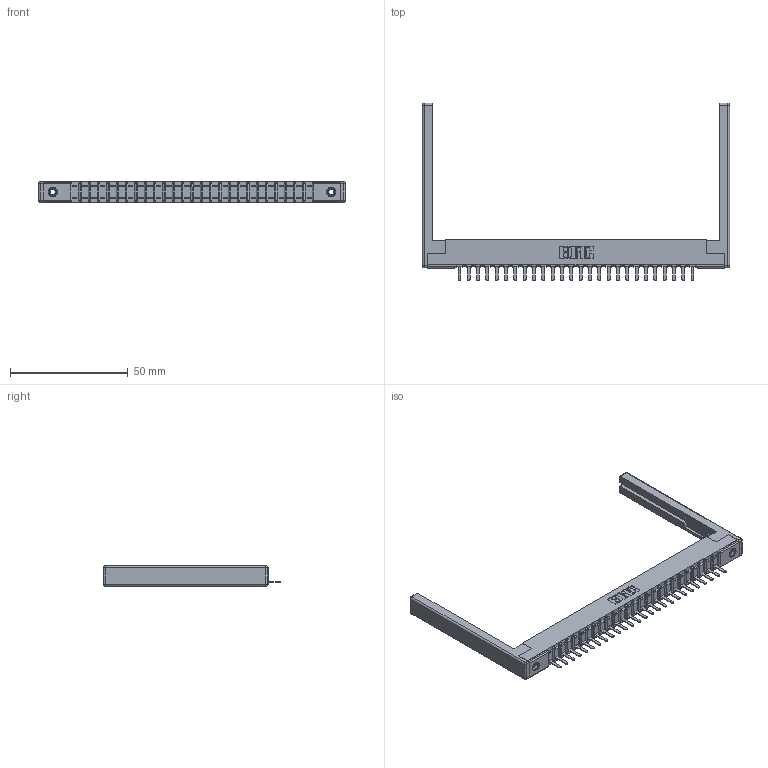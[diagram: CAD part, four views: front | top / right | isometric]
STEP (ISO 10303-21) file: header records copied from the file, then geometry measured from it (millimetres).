
FILE_DESCRIPTION (( 'STEP AP203' ), '1' );
FILE_NAME ('357-026-521-168.STEP', '2019-09-17T01:04:23', ( '' ), ( '' ), 'SwSTEP 2.0', 'SolidWorks 2016', '' );
FILE_SCHEMA (( 'CONFIG_CONTROL_DESIGN' ));
Length unit declared in the file: inch
Products named in the file (5): 307-290-002_521; 307 Part_.156 Dia Mounting Holes; 357-026-521-168; 307-220-068; 345-250-001_345-250-001-102
Assembly tree (31 placements, depth 2):
  357-026-521-168
    307 Part_.156 Dia Mounting Holes
    307-290-002_521  x26
    307-220-068  x2
    345-250-001_345-250-001-102  x2
Bounding box: 130.45 x 75.39 x 8.71 mm (x, y, z)
Volume: 13174.8 mm3; surface area: 19929.5 mm2
Topology: 31 solids, 31 shells, 2223 faces, 6745 edges, 4402 vertices
Faces by surface type: plane 1328, cylinder 817, sphere 62, cone 12, torus 4
Entity records: 27739 total; most frequent: CARTESIAN_POINT 4641, ORIENTED_EDGE 4620, DIRECTION 4534, EDGE_CURVE 2310, VECTOR 1760, LINE 1760, VERTEX_POINT 1494, AXIS2_PLACEMENT_3D 1387
